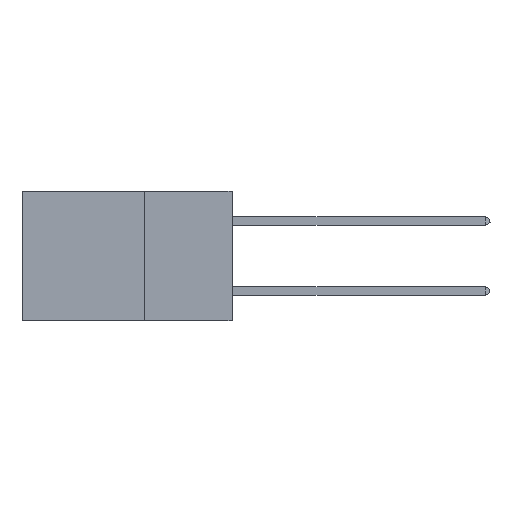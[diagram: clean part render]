
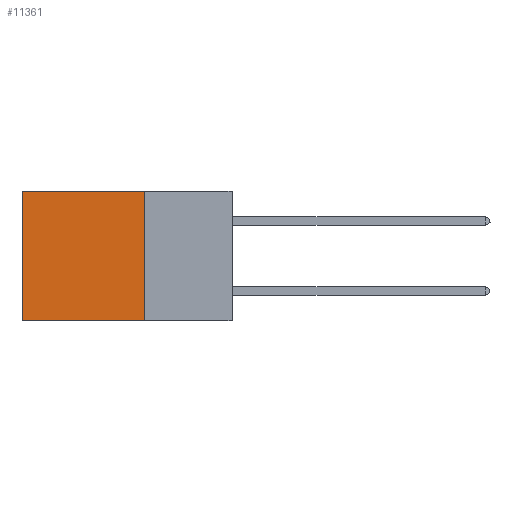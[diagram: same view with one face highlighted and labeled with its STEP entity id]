
A CAD part, left-side view. The second image highlights one B-rep face of the part: STEP entity #11361.
In plain terms, the highlighted planar face has unit normal (-1, 0, 0).
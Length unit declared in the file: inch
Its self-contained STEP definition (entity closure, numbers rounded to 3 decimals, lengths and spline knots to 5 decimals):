
#1778 = CARTESIAN_POINT ( 'NONE',  ( 0.2875, 0.25, 0. ) ) ;
#2031 = VECTOR ( 'NONE', #9899, 39.37008 ) ;
#2707 = CARTESIAN_POINT ( 'NONE',  ( 0.2875, 0.25, 0. ) ) ;
#2822 = LINE ( 'NONE', #4421, #10182 ) ;
#2846 = FACE_OUTER_BOUND ( 'NONE', #16561, .T. ) ;
#3158 = ORIENTED_EDGE ( 'NONE', *, *, #6208, .F. ) ;
#3178 = ORIENTED_EDGE ( 'NONE', *, *, #5133, .T. ) ;
#3662 = DIRECTION ( 'NONE',  ( 0., 0., -1. ) ) ;
#4054 = EDGE_CURVE ( 'NONE', #12241, #18954, #2822, .T. ) ;
#4421 = CARTESIAN_POINT ( 'NONE',  ( 0.2875, 0.25, 0. ) ) ;
#5133 = EDGE_CURVE ( 'NONE', #18954, #7075, #12753, .T. ) ;
#5996 = DIRECTION ( 'NONE',  ( 0., 1., 0. ) ) ;
#6208 = EDGE_CURVE ( 'NONE', #15261, #7075, #8291, .T. ) ;
#6793 = CARTESIAN_POINT ( 'NONE',  ( 0.2875, 0.25, -0.37 ) ) ;
#6950 = CARTESIAN_POINT ( 'NONE',  ( 0.2875, 0.6, 0. ) ) ;
#7075 = VERTEX_POINT ( 'NONE', #15832 ) ;
#7225 = CARTESIAN_POINT ( 'NONE',  ( 0.2875, 0.25, -0.37 ) ) ;
#7529 = PLANE ( 'NONE',  #19586 ) ;
#7951 = EDGE_CURVE ( 'NONE', #12241, #15261, #13893, .T. ) ;
#8291 = LINE ( 'NONE', #6793, #2031 ) ;
#8851 = DIRECTION ( 'NONE',  ( 0., 0., -1. ) ) ;
#9899 = DIRECTION ( 'NONE',  ( 0., 1., 0. ) ) ;
#10182 = VECTOR ( 'NONE', #5996, 39.37008 ) ;
#10655 = ORIENTED_EDGE ( 'NONE', *, *, #4054, .T. ) ;
#11361 = ADVANCED_FACE ( 'NONE', ( #2846 ), #7529, .F. ) ;
#12241 = VERTEX_POINT ( 'NONE', #2707 ) ;
#12296 = DIRECTION ( 'NONE',  ( 0., 0., -1. ) ) ;
#12753 = LINE ( 'NONE', #6950, #18213 ) ;
#13829 = CARTESIAN_POINT ( 'NONE',  ( 0.2875, 0.25, 0. ) ) ;
#13893 = LINE ( 'NONE', #1778, #14220 ) ;
#14220 = VECTOR ( 'NONE', #12296, 39.37008 ) ;
#15038 = DIRECTION ( 'NONE',  ( 1., 0., 0. ) ) ;
#15261 = VERTEX_POINT ( 'NONE', #7225 ) ;
#15832 = CARTESIAN_POINT ( 'NONE',  ( 0.2875, 0.6, -0.37 ) ) ;
#16561 = EDGE_LOOP ( 'NONE', ( #3178, #3158, #19459, #10655 ) ) ;
#17071 = CARTESIAN_POINT ( 'NONE',  ( 0.2875, 0.6, 0. ) ) ;
#18213 = VECTOR ( 'NONE', #3662, 39.37008 ) ;
#18954 = VERTEX_POINT ( 'NONE', #17071 ) ;
#19459 = ORIENTED_EDGE ( 'NONE', *, *, #7951, .F. ) ;
#19586 = AXIS2_PLACEMENT_3D ( 'NONE', #13829, #15038, #8851 ) ;
